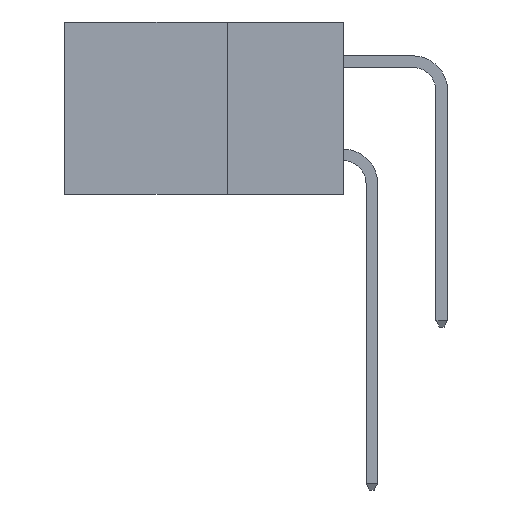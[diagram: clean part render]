
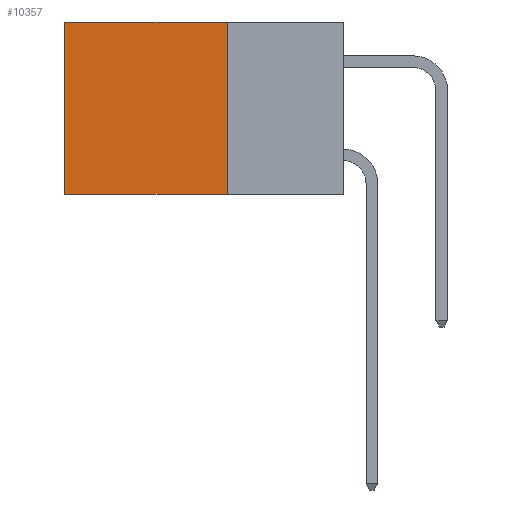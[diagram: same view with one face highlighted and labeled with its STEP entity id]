
A CAD part, left-side view. The second image highlights one B-rep face of the part: STEP entity #10357.
In plain terms, the highlighted planar face has unit normal (-1, 0, 0).
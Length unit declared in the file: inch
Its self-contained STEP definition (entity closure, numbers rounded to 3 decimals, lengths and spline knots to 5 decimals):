
#458 = VERTEX_POINT ( 'NONE', #2798 ) ;
#525 = DIRECTION ( 'NONE',  ( 0., 0., -1. ) ) ;
#710 = ORIENTED_EDGE ( 'NONE', *, *, #8682, .T. ) ;
#892 = LINE ( 'NONE', #14481, #9137 ) ;
#1172 = LINE ( 'NONE', #9200, #17196 ) ;
#1284 = VERTEX_POINT ( 'NONE', #9743 ) ;
#1670 = AXIS2_PLACEMENT_3D ( 'NONE', #2382, #13609, #4025 ) ;
#1952 = EDGE_CURVE ( 'NONE', #6088, #1284, #892, .T. ) ;
#1961 = VERTEX_POINT ( 'NONE', #15767 ) ;
#2382 = CARTESIAN_POINT ( 'NONE',  ( 0.2615, 0.25, -0.37 ) ) ;
#2798 = CARTESIAN_POINT ( 'NONE',  ( 0.2615, 0.25, -0.37 ) ) ;
#3861 = CARTESIAN_POINT ( 'NONE',  ( 0.2615, 0.25, -0.37 ) ) ;
#4025 = DIRECTION ( 'NONE',  ( 0., 0., -1. ) ) ;
#4322 = DIRECTION ( 'NONE',  ( 0., 1., 0. ) ) ;
#4673 = FACE_OUTER_BOUND ( 'NONE', #16353, .T. ) ;
#5821 = ORIENTED_EDGE ( 'NONE', *, *, #1952, .T. ) ;
#5871 = ORIENTED_EDGE ( 'NONE', *, *, #20579, .F. ) ;
#6088 = VERTEX_POINT ( 'NONE', #18840 ) ;
#6090 = CARTESIAN_POINT ( 'NONE',  ( 0.2615, 0.6, -0.37 ) ) ;
#7777 = EDGE_CURVE ( 'NONE', #458, #1961, #1172, .T. ) ;
#8682 = EDGE_CURVE ( 'NONE', #1284, #1961, #9369, .T. ) ;
#9137 = VECTOR ( 'NONE', #14628, 39.37008 ) ;
#9200 = CARTESIAN_POINT ( 'NONE',  ( 0.2615, 0.25, -0.37 ) ) ;
#9369 = LINE ( 'NONE', #6090, #17637 ) ;
#9743 = CARTESIAN_POINT ( 'NONE',  ( 0.2615, 0.6, 0. ) ) ;
#10357 = ADVANCED_FACE ( 'NONE', ( #4673 ), #15127, .F. ) ;
#11018 = DIRECTION ( 'NONE',  ( 0., 0., -1. ) ) ;
#13261 = VECTOR ( 'NONE', #525, 39.37008 ) ;
#13609 = DIRECTION ( 'NONE',  ( 1., 0., 0. ) ) ;
#13750 = LINE ( 'NONE', #3861, #13261 ) ;
#14481 = CARTESIAN_POINT ( 'NONE',  ( 0.2615, 0.25, 0. ) ) ;
#14628 = DIRECTION ( 'NONE',  ( 0., 1., 0. ) ) ;
#15127 = PLANE ( 'NONE',  #1670 ) ;
#15675 = ORIENTED_EDGE ( 'NONE', *, *, #7777, .F. ) ;
#15767 = CARTESIAN_POINT ( 'NONE',  ( 0.2615, 0.6, -0.37 ) ) ;
#16353 = EDGE_LOOP ( 'NONE', ( #710, #15675, #5871, #5821 ) ) ;
#17196 = VECTOR ( 'NONE', #4322, 39.37008 ) ;
#17637 = VECTOR ( 'NONE', #11018, 39.37008 ) ;
#18840 = CARTESIAN_POINT ( 'NONE',  ( 0.2615, 0.25, 0. ) ) ;
#20579 = EDGE_CURVE ( 'NONE', #6088, #458, #13750, .T. ) ;
